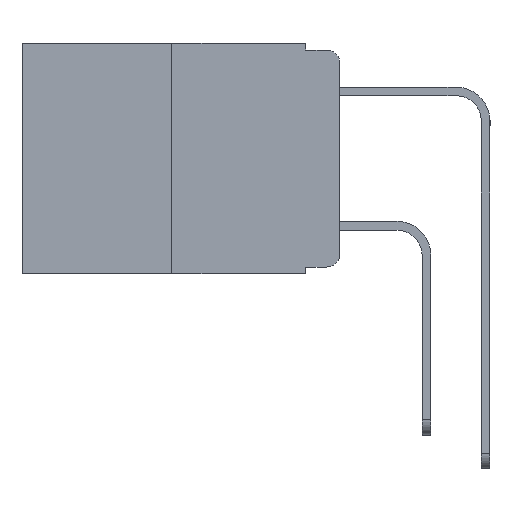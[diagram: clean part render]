
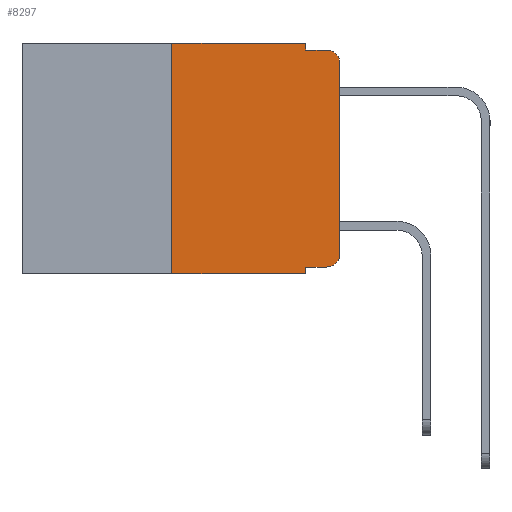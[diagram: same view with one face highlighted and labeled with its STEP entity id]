
A CAD part, left-side view. The second image highlights one B-rep face of the part: STEP entity #8297.
In plain terms, the highlighted planar face has unit normal (-1, 0, 0).
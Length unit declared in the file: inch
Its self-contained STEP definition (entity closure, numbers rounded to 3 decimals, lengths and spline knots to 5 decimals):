
#292 = CIRCLE ( 'NONE', #8337, 0.02 ) ;
#309 = CARTESIAN_POINT ( 'NONE',  ( 0., 0., -0.313 ) ) ;
#594 = EDGE_CURVE ( 'NONE', #1548, #7635, #2854, .T. ) ;
#672 = EDGE_CURVE ( 'NONE', #11372, #13141, #7352, .T. ) ;
#685 = DIRECTION ( 'NONE',  ( 1., 0., 0. ) ) ;
#786 = ORIENTED_EDGE ( 'NONE', *, *, #3256, .F. ) ;
#795 = ORIENTED_EDGE ( 'NONE', *, *, #594, .T. ) ;
#1184 = VERTEX_POINT ( 'NONE', #12559 ) ;
#1439 = VECTOR ( 'NONE', #10650, 39.37008 ) ;
#1479 = CARTESIAN_POINT ( 'NONE',  ( 0., 0.051, -0.343 ) ) ;
#1547 = VERTEX_POINT ( 'NONE', #9084 ) ;
#1548 = VERTEX_POINT ( 'NONE', #7427 ) ;
#1585 = EDGE_CURVE ( 'NONE', #1184, #1547, #5522, .T. ) ;
#1703 = VERTEX_POINT ( 'NONE', #4763 ) ;
#1948 = CARTESIAN_POINT ( 'NONE',  ( 0., 0.051, -0.333 ) ) ;
#1990 = LINE ( 'NONE', #3660, #2652 ) ;
#2096 = VECTOR ( 'NONE', #13262, 39.37008 ) ;
#2635 = ORIENTED_EDGE ( 'NONE', *, *, #4856, .F. ) ;
#2652 = VECTOR ( 'NONE', #8634, 39.37008 ) ;
#2837 = EDGE_CURVE ( 'NONE', #9003, #1547, #292, .T. ) ;
#2854 = CIRCLE ( 'NONE', #6057, 0.02 ) ;
#2860 = VECTOR ( 'NONE', #12215, 39.37008 ) ;
#2982 = ORIENTED_EDGE ( 'NONE', *, *, #4606, .F. ) ;
#3025 = CARTESIAN_POINT ( 'NONE',  ( 0., 0.25, 0. ) ) ;
#3256 = EDGE_CURVE ( 'NONE', #13141, #1184, #1990, .T. ) ;
#3347 = VERTEX_POINT ( 'NONE', #6142 ) ;
#3660 = CARTESIAN_POINT ( 'NONE',  ( 0., 0.051, 0. ) ) ;
#3917 = ORIENTED_EDGE ( 'NONE', *, *, #11102, .T. ) ;
#3950 = CARTESIAN_POINT ( 'NONE',  ( 0., 0.02, -0.03 ) ) ;
#4216 = LINE ( 'NONE', #4231, #1439 ) ;
#4231 = CARTESIAN_POINT ( 'NONE',  ( 0., 0.25, 0. ) ) ;
#4452 = VERTEX_POINT ( 'NONE', #1479 ) ;
#4606 = EDGE_CURVE ( 'NONE', #3347, #4452, #6479, .T. ) ;
#4741 = VECTOR ( 'NONE', #11713, 39.37008 ) ;
#4763 = CARTESIAN_POINT ( 'NONE',  ( 0., 0.25, -0.343 ) ) ;
#4808 = LINE ( 'NONE', #12844, #2096 ) ;
#4856 = EDGE_CURVE ( 'NONE', #1703, #11372, #4216, .T. ) ;
#4908 = DIRECTION ( 'NONE',  ( 0., -1., 0. ) ) ;
#5522 = LINE ( 'NONE', #6869, #8010 ) ;
#5530 = LINE ( 'NONE', #1948, #2860 ) ;
#5650 = ORIENTED_EDGE ( 'NONE', *, *, #672, .F. ) ;
#6057 = AXIS2_PLACEMENT_3D ( 'NONE', #8718, #6452, #12054 ) ;
#6121 = EDGE_CURVE ( 'NONE', #1703, #4452, #4808, .T. ) ;
#6142 = CARTESIAN_POINT ( 'NONE',  ( 0., 0.051, -0.333 ) ) ;
#6347 = CARTESIAN_POINT ( 'NONE',  ( 0., 0., -0.03 ) ) ;
#6452 = DIRECTION ( 'NONE',  ( -1., 0., 0. ) ) ;
#6479 = LINE ( 'NONE', #12856, #11621 ) ;
#6869 = CARTESIAN_POINT ( 'NONE',  ( 0., 0.051, -0.01 ) ) ;
#7009 = ORIENTED_EDGE ( 'NONE', *, *, #10848, .T. ) ;
#7038 = ORIENTED_EDGE ( 'NONE', *, *, #1585, .F. ) ;
#7109 = DIRECTION ( 'NONE',  ( 0., -1., 0. ) ) ;
#7352 = LINE ( 'NONE', #8739, #12792 ) ;
#7427 = CARTESIAN_POINT ( 'NONE',  ( 0., 0.02, -0.333 ) ) ;
#7635 = VERTEX_POINT ( 'NONE', #309 ) ;
#7838 = LINE ( 'NONE', #12681, #4741 ) ;
#7965 = DIRECTION ( 'NONE',  ( 0., 0., -1. ) ) ;
#8010 = VECTOR ( 'NONE', #7109, 39.37008 ) ;
#8188 = DIRECTION ( 'NONE',  ( -1., 0., 0. ) ) ;
#8297 = ADVANCED_FACE ( 'NONE', ( #13332 ), #13057, .F. ) ;
#8337 = AXIS2_PLACEMENT_3D ( 'NONE', #3950, #8188, #12982 ) ;
#8634 = DIRECTION ( 'NONE',  ( 0., 0., -1. ) ) ;
#8718 = CARTESIAN_POINT ( 'NONE',  ( 0., 0.02, -0.313 ) ) ;
#8739 = CARTESIAN_POINT ( 'NONE',  ( 0., 0.473, 0. ) ) ;
#9003 = VERTEX_POINT ( 'NONE', #6347 ) ;
#9020 = ORIENTED_EDGE ( 'NONE', *, *, #2837, .T. ) ;
#9084 = CARTESIAN_POINT ( 'NONE',  ( 0., 0.02, -0.01 ) ) ;
#10650 = DIRECTION ( 'NONE',  ( 0., 0., 1. ) ) ;
#10848 = EDGE_CURVE ( 'NONE', #3347, #1548, #5530, .T. ) ;
#10872 = CARTESIAN_POINT ( 'NONE',  ( 0., 0.051, 0. ) ) ;
#10974 = CARTESIAN_POINT ( 'NONE',  ( 0., 0.473, 0. ) ) ;
#11102 = EDGE_CURVE ( 'NONE', #7635, #9003, #7838, .T. ) ;
#11359 = ORIENTED_EDGE ( 'NONE', *, *, #6121, .T. ) ;
#11372 = VERTEX_POINT ( 'NONE', #3025 ) ;
#11503 = EDGE_LOOP ( 'NONE', ( #3917, #9020, #7038, #786, #5650, #2635, #11359, #2982, #7009, #795 ) ) ;
#11621 = VECTOR ( 'NONE', #12166, 39.37008 ) ;
#11713 = DIRECTION ( 'NONE',  ( 0., 0., 1. ) ) ;
#12054 = DIRECTION ( 'NONE',  ( 0., 0., -1. ) ) ;
#12159 = AXIS2_PLACEMENT_3D ( 'NONE', #10974, #685, #7965 ) ;
#12166 = DIRECTION ( 'NONE',  ( 0., 0., -1. ) ) ;
#12215 = DIRECTION ( 'NONE',  ( 0., -1., 0. ) ) ;
#12559 = CARTESIAN_POINT ( 'NONE',  ( 0., 0.051, -0.01 ) ) ;
#12681 = CARTESIAN_POINT ( 'NONE',  ( 0., 0., 0. ) ) ;
#12792 = VECTOR ( 'NONE', #4908, 39.37008 ) ;
#12844 = CARTESIAN_POINT ( 'NONE',  ( 0., 0.473, -0.343 ) ) ;
#12856 = CARTESIAN_POINT ( 'NONE',  ( 0., 0.051, 0. ) ) ;
#12982 = DIRECTION ( 'NONE',  ( 0., 0., -1. ) ) ;
#13057 = PLANE ( 'NONE',  #12159 ) ;
#13141 = VERTEX_POINT ( 'NONE', #10872 ) ;
#13262 = DIRECTION ( 'NONE',  ( 0., -1., 0. ) ) ;
#13332 = FACE_OUTER_BOUND ( 'NONE', #11503, .T. ) ;
